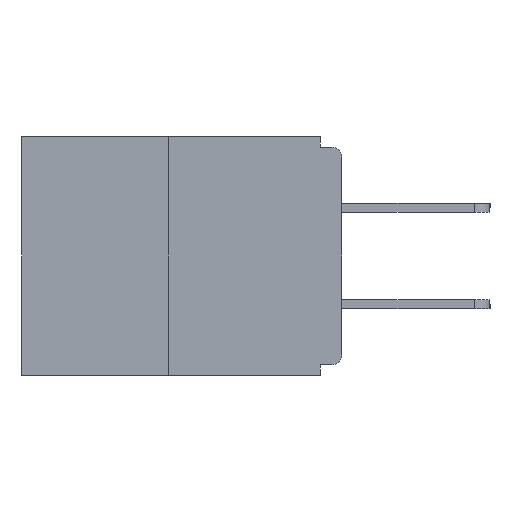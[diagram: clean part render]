
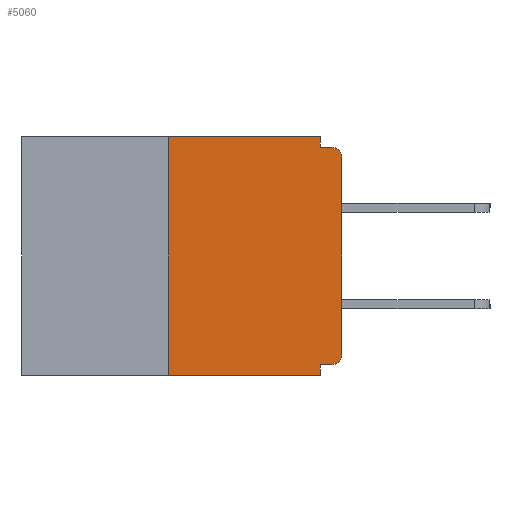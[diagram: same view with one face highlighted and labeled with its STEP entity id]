
A CAD part, left-side view. The second image highlights one B-rep face of the part: STEP entity #5060.
In plain terms, the highlighted planar face has unit normal (-1, 0, 0).
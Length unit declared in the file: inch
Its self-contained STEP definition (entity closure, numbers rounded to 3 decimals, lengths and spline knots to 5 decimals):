
#42 = VECTOR ( 'NONE', #13351, 39.37008 ) ;
#176 = VECTOR ( 'NONE', #2725, 39.37008 ) ;
#300 = VECTOR ( 'NONE', #15250, 39.37008 ) ;
#492 = EDGE_CURVE ( 'NONE', #9467, #9415, #10848, .T. ) ;
#697 = DIRECTION ( 'NONE',  ( 0., 0., -1. ) ) ;
#765 = CARTESIAN_POINT ( 'NONE',  ( 0., 0.015, -0.313 ) ) ;
#813 = DIRECTION ( 'NONE',  ( 0., 0., -1. ) ) ;
#849 = DIRECTION ( 'NONE',  ( 0., 1., 0. ) ) ;
#1112 = LINE ( 'NONE', #2069, #12606 ) ;
#1156 = CARTESIAN_POINT ( 'NONE',  ( 0., 0.031, -0.015 ) ) ;
#1176 = DIRECTION ( 'NONE',  ( 0., 0., -1. ) ) ;
#1187 = VERTEX_POINT ( 'NONE', #18974 ) ;
#1202 = CARTESIAN_POINT ( 'NONE',  ( 0., 0., 0. ) ) ;
#1226 = VERTEX_POINT ( 'NONE', #2398 ) ;
#1881 = CARTESIAN_POINT ( 'NONE',  ( 0., 0.25, 0. ) ) ;
#1975 = CARTESIAN_POINT ( 'NONE',  ( 0., 0.015, -0.015 ) ) ;
#2069 = CARTESIAN_POINT ( 'NONE',  ( 0., 0., -0.015 ) ) ;
#2173 = ORIENTED_EDGE ( 'NONE', *, *, #2787, .F. ) ;
#2398 = CARTESIAN_POINT ( 'NONE',  ( 0., 0.031, 0. ) ) ;
#2648 = VERTEX_POINT ( 'NONE', #7883 ) ;
#2725 = DIRECTION ( 'NONE',  ( 0., -1., 0. ) ) ;
#2782 = LINE ( 'NONE', #14276, #6749 ) ;
#2787 = EDGE_CURVE ( 'NONE', #2648, #13340, #16389, .T. ) ;
#2977 = CARTESIAN_POINT ( 'NONE',  ( 0., 0.46, 0. ) ) ;
#3276 = ORIENTED_EDGE ( 'NONE', *, *, #492, .T. ) ;
#3359 = CARTESIAN_POINT ( 'NONE',  ( 0., 0., -0.313 ) ) ;
#3692 = CARTESIAN_POINT ( 'NONE',  ( 0., 0.015, -0.03 ) ) ;
#3803 = DIRECTION ( 'NONE',  ( 0., 0., -1. ) ) ;
#4226 = ORIENTED_EDGE ( 'NONE', *, *, #18071, .F. ) ;
#4337 = VERTEX_POINT ( 'NONE', #1975 ) ;
#4553 = DIRECTION ( 'NONE',  ( 1., 0., 0. ) ) ;
#4855 = CARTESIAN_POINT ( 'NONE',  ( 0., 0., -0.03 ) ) ;
#4950 = ORIENTED_EDGE ( 'NONE', *, *, #10231, .T. ) ;
#5060 = ADVANCED_FACE ( 'NONE', ( #14755 ), #6115, .F. ) ;
#5384 = CARTESIAN_POINT ( 'NONE',  ( 0., 0.031, -0.343 ) ) ;
#5472 = ORIENTED_EDGE ( 'NONE', *, *, #9133, .T. ) ;
#5600 = EDGE_CURVE ( 'NONE', #18636, #2648, #2782, .T. ) ;
#5923 = DIRECTION ( 'NONE',  ( 0., 0., 1. ) ) ;
#6115 = PLANE ( 'NONE',  #18168 ) ;
#6138 = EDGE_CURVE ( 'NONE', #18636, #9467, #11662, .T. ) ;
#6148 = ORIENTED_EDGE ( 'NONE', *, *, #5600, .F. ) ;
#6663 = ORIENTED_EDGE ( 'NONE', *, *, #6138, .T. ) ;
#6749 = VECTOR ( 'NONE', #849, 39.37008 ) ;
#7126 = CARTESIAN_POINT ( 'NONE',  ( 0., 0.46, 0. ) ) ;
#7496 = DIRECTION ( 'NONE',  ( 0., 0., -1. ) ) ;
#7583 = CIRCLE ( 'NONE', #16240, 0.015 ) ;
#7680 = VECTOR ( 'NONE', #1176, 39.37008 ) ;
#7883 = CARTESIAN_POINT ( 'NONE',  ( 0., 0.031, -0.328 ) ) ;
#8103 = EDGE_LOOP ( 'NONE', ( #11004, #12443, #4950, #2173, #6148, #6663, #3276, #5472, #4226, #16779 ) ) ;
#8167 = DIRECTION ( 'NONE',  ( -1., 0., 0. ) ) ;
#9133 = EDGE_CURVE ( 'NONE', #9415, #4337, #7583, .T. ) ;
#9415 = VERTEX_POINT ( 'NONE', #4855 ) ;
#9467 = VERTEX_POINT ( 'NONE', #3359 ) ;
#9885 = EDGE_CURVE ( 'NONE', #11378, #1187, #15513, .T. ) ;
#10231 = EDGE_CURVE ( 'NONE', #11378, #13340, #12670, .T. ) ;
#10248 = VERTEX_POINT ( 'NONE', #1156 ) ;
#10848 = LINE ( 'NONE', #1202, #18800 ) ;
#11004 = ORIENTED_EDGE ( 'NONE', *, *, #18914, .F. ) ;
#11378 = VERTEX_POINT ( 'NONE', #13258 ) ;
#11516 = EDGE_CURVE ( 'NONE', #1226, #10248, #17307, .T. ) ;
#11662 = CIRCLE ( 'NONE', #15769, 0.015 ) ;
#11912 = VECTOR ( 'NONE', #813, 39.37008 ) ;
#12443 = ORIENTED_EDGE ( 'NONE', *, *, #9885, .F. ) ;
#12563 = DIRECTION ( 'NONE',  ( 0., -1., 0. ) ) ;
#12606 = VECTOR ( 'NONE', #12563, 39.37008 ) ;
#12670 = LINE ( 'NONE', #19255, #42 ) ;
#12740 = DIRECTION ( 'NONE',  ( -1., 0., 0. ) ) ;
#12785 = CARTESIAN_POINT ( 'NONE',  ( 0., 0.031, -0.343 ) ) ;
#13258 = CARTESIAN_POINT ( 'NONE',  ( 0., 0.25, -0.343 ) ) ;
#13340 = VERTEX_POINT ( 'NONE', #5384 ) ;
#13351 = DIRECTION ( 'NONE',  ( 0., -1., 0. ) ) ;
#14276 = CARTESIAN_POINT ( 'NONE',  ( 0., 0., -0.328 ) ) ;
#14755 = FACE_OUTER_BOUND ( 'NONE', #8103, .T. ) ;
#15250 = DIRECTION ( 'NONE',  ( 0., 0., 1. ) ) ;
#15513 = LINE ( 'NONE', #1881, #300 ) ;
#15769 = AXIS2_PLACEMENT_3D ( 'NONE', #765, #12740, #3803 ) ;
#16240 = AXIS2_PLACEMENT_3D ( 'NONE', #3692, #8167, #697 ) ;
#16342 = CARTESIAN_POINT ( 'NONE',  ( 0., 0.031, 0. ) ) ;
#16356 = LINE ( 'NONE', #7126, #176 ) ;
#16389 = LINE ( 'NONE', #12785, #11912 ) ;
#16779 = ORIENTED_EDGE ( 'NONE', *, *, #11516, .F. ) ;
#17307 = LINE ( 'NONE', #16342, #7680 ) ;
#18071 = EDGE_CURVE ( 'NONE', #10248, #4337, #1112, .T. ) ;
#18168 = AXIS2_PLACEMENT_3D ( 'NONE', #2977, #4553, #7496 ) ;
#18636 = VERTEX_POINT ( 'NONE', #19290 ) ;
#18800 = VECTOR ( 'NONE', #5923, 39.37008 ) ;
#18914 = EDGE_CURVE ( 'NONE', #1187, #1226, #16356, .T. ) ;
#18974 = CARTESIAN_POINT ( 'NONE',  ( 0., 0.25, 0. ) ) ;
#19255 = CARTESIAN_POINT ( 'NONE',  ( 0., 0.46, -0.343 ) ) ;
#19290 = CARTESIAN_POINT ( 'NONE',  ( 0., 0.015, -0.328 ) ) ;
